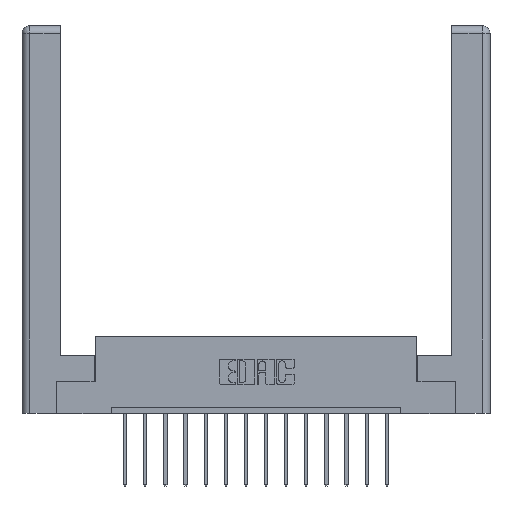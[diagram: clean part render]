
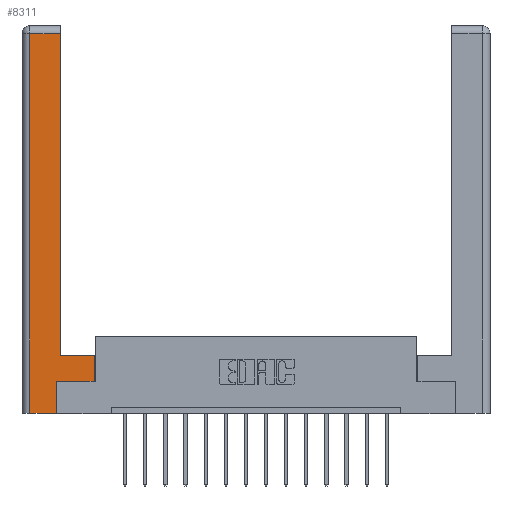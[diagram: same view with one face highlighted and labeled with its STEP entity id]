
A CAD part, top view. The second image highlights one B-rep face of the part: STEP entity #8311.
In plain terms, the highlighted planar face has unit normal (0, 0, 1).
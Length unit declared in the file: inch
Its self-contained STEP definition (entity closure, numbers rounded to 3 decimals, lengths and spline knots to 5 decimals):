
#9 = LINE ( 'NONE', #7228, #2235 ) ;
#362 = EDGE_LOOP ( 'NONE', ( #12417, #11522, #422, #11192, #12340, #14260, #3607, #14576 ) ) ;
#422 = ORIENTED_EDGE ( 'NONE', *, *, #14942, .T. ) ;
#785 = DIRECTION ( 'NONE',  ( 0., 1., 0. ) ) ;
#1147 = CARTESIAN_POINT ( 'NONE',  ( 0.0615, 0., 0. ) ) ;
#1203 = LINE ( 'NONE', #6622, #2614 ) ;
#1257 = LINE ( 'NONE', #10057, #8528 ) ;
#1329 = VECTOR ( 'NONE', #1849, 39.37008 ) ;
#1387 = DIRECTION ( 'NONE',  ( 1., 0., 0. ) ) ;
#1578 = CARTESIAN_POINT ( 'NONE',  ( 0.295, 2.94, 0. ) ) ;
#1849 = DIRECTION ( 'NONE',  ( 0., 1., 0. ) ) ;
#1921 = EDGE_CURVE ( 'NONE', #15053, #10098, #9613, .T. ) ;
#2039 = LINE ( 'NONE', #11167, #3659 ) ;
#2232 = CARTESIAN_POINT ( 'NONE',  ( 0.265, 0.245, 0. ) ) ;
#2235 = VECTOR ( 'NONE', #16345, 39.37008 ) ;
#2523 = EDGE_CURVE ( 'NONE', #10098, #11205, #7151, .T. ) ;
#2614 = VECTOR ( 'NONE', #15513, 39.37008 ) ;
#2883 = CARTESIAN_POINT ( 'NONE',  ( 0.0615, 0., 0. ) ) ;
#3054 = CARTESIAN_POINT ( 'NONE',  ( 0.0615, 2.94, 0. ) ) ;
#3083 = CARTESIAN_POINT ( 'NONE',  ( 0.265, 0., 0. ) ) ;
#3512 = VECTOR ( 'NONE', #7357, 39.37008 ) ;
#3607 = ORIENTED_EDGE ( 'NONE', *, *, #11350, .T. ) ;
#3659 = VECTOR ( 'NONE', #785, 39.37008 ) ;
#3668 = VERTEX_POINT ( 'NONE', #3083 ) ;
#4117 = EDGE_CURVE ( 'NONE', #15771, #14092, #10906, .T. ) ;
#4209 = VERTEX_POINT ( 'NONE', #8199 ) ;
#4506 = EDGE_CURVE ( 'NONE', #4209, #15053, #1203, .T. ) ;
#5227 = VECTOR ( 'NONE', #1387, 39.37008 ) ;
#6622 = CARTESIAN_POINT ( 'NONE',  ( 0.295, 0.45, 0. ) ) ;
#7151 = LINE ( 'NONE', #9959, #3512 ) ;
#7228 = CARTESIAN_POINT ( 'NONE',  ( 0.265, 0.245, 0. ) ) ;
#7328 = LINE ( 'NONE', #2883, #16165 ) ;
#7357 = DIRECTION ( 'NONE',  ( -1., 0., 0. ) ) ;
#7573 = DIRECTION ( 'NONE',  ( 1., 0., 0. ) ) ;
#7641 = CARTESIAN_POINT ( 'NONE',  ( 0.565, 0.245, 0. ) ) ;
#8199 = CARTESIAN_POINT ( 'NONE',  ( 0.565, 0.45, 0. ) ) ;
#8311 = ADVANCED_FACE ( 'NONE', ( #15588 ), #15392, .F. ) ;
#8528 = VECTOR ( 'NONE', #7573, 39.37008 ) ;
#9126 = VERTEX_POINT ( 'NONE', #1147 ) ;
#9613 = LINE ( 'NONE', #14914, #1329 ) ;
#9758 = EDGE_CURVE ( 'NONE', #3668, #15771, #9, .T. ) ;
#9959 = CARTESIAN_POINT ( 'NONE',  ( 0.0615, 2.94, 0. ) ) ;
#10057 = CARTESIAN_POINT ( 'NONE',  ( 0.265, 0., 0. ) ) ;
#10098 = VERTEX_POINT ( 'NONE', #1578 ) ;
#10906 = LINE ( 'NONE', #15352, #5227 ) ;
#10936 = EDGE_CURVE ( 'NONE', #9126, #3668, #1257, .T. ) ;
#11167 = CARTESIAN_POINT ( 'NONE',  ( 0.565, 0.45, 0. ) ) ;
#11192 = ORIENTED_EDGE ( 'NONE', *, *, #10936, .T. ) ;
#11205 = VERTEX_POINT ( 'NONE', #3054 ) ;
#11350 = EDGE_CURVE ( 'NONE', #14092, #4209, #2039, .T. ) ;
#11522 = ORIENTED_EDGE ( 'NONE', *, *, #2523, .T. ) ;
#11614 = CARTESIAN_POINT ( 'NONE',  ( 0., 0., 0. ) ) ;
#12172 = AXIS2_PLACEMENT_3D ( 'NONE', #11614, #14159, #14324 ) ;
#12340 = ORIENTED_EDGE ( 'NONE', *, *, #9758, .T. ) ;
#12417 = ORIENTED_EDGE ( 'NONE', *, *, #1921, .T. ) ;
#14092 = VERTEX_POINT ( 'NONE', #7641 ) ;
#14159 = DIRECTION ( 'NONE',  ( 0., 0., -1. ) ) ;
#14260 = ORIENTED_EDGE ( 'NONE', *, *, #4117, .T. ) ;
#14324 = DIRECTION ( 'NONE',  ( -1., 0., 0. ) ) ;
#14493 = DIRECTION ( 'NONE',  ( 0., -1., 0. ) ) ;
#14576 = ORIENTED_EDGE ( 'NONE', *, *, #4506, .T. ) ;
#14914 = CARTESIAN_POINT ( 'NONE',  ( 0.295, 3., 0. ) ) ;
#14942 = EDGE_CURVE ( 'NONE', #11205, #9126, #7328, .T. ) ;
#15053 = VERTEX_POINT ( 'NONE', #15997 ) ;
#15352 = CARTESIAN_POINT ( 'NONE',  ( 0.565, 0.245, 0. ) ) ;
#15392 = PLANE ( 'NONE',  #12172 ) ;
#15513 = DIRECTION ( 'NONE',  ( -1., 0., 0. ) ) ;
#15588 = FACE_OUTER_BOUND ( 'NONE', #362, .T. ) ;
#15771 = VERTEX_POINT ( 'NONE', #2232 ) ;
#15997 = CARTESIAN_POINT ( 'NONE',  ( 0.295, 0.45, 0. ) ) ;
#16165 = VECTOR ( 'NONE', #14493, 39.37008 ) ;
#16345 = DIRECTION ( 'NONE',  ( 0., 1., 0. ) ) ;
